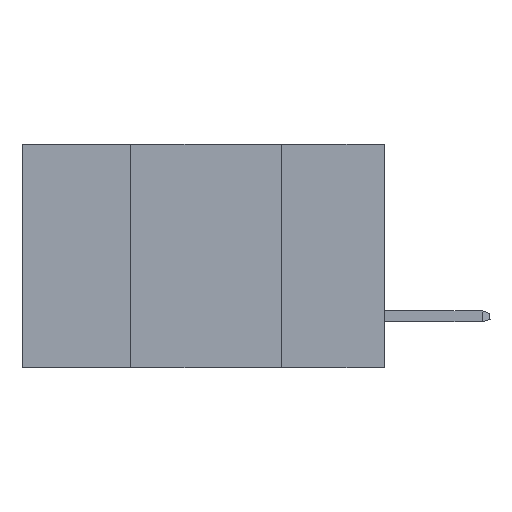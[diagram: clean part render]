
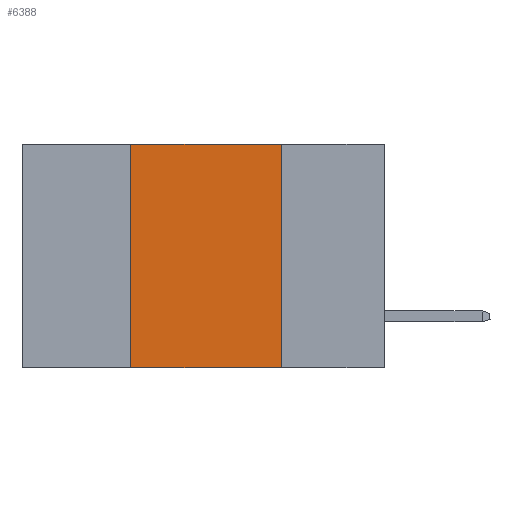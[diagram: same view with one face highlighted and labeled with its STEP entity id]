
A CAD part, left-side view. The second image highlights one B-rep face of the part: STEP entity #6388.
In plain terms, the highlighted planar face has unit normal (-1, 0, 0).
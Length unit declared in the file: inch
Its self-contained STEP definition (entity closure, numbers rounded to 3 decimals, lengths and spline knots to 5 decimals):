
#297 = VERTEX_POINT ( 'NONE', #6167 ) ;
#317 = LINE ( 'NONE', #12907, #29280 ) ;
#359 = DIRECTION ( 'NONE',  ( 0., 0., -1. ) ) ;
#3723 = EDGE_CURVE ( 'NONE', #297, #7186, #22911, .T. ) ;
#4326 = LINE ( 'NONE', #20937, #27781 ) ;
#5648 = ORIENTED_EDGE ( 'NONE', *, *, #17468, .F. ) ;
#5982 = ORIENTED_EDGE ( 'NONE', *, *, #3723, .F. ) ;
#6167 = CARTESIAN_POINT ( 'NONE',  ( 0., 0.42, 0. ) ) ;
#6230 = CARTESIAN_POINT ( 'NONE',  ( 0., 0.17, 0. ) ) ;
#6388 = ADVANCED_FACE ( 'NONE', ( #8823 ), #24045, .F. ) ;
#6998 = CARTESIAN_POINT ( 'NONE',  ( 0., 0.42, 0. ) ) ;
#7186 = VERTEX_POINT ( 'NONE', #6230 ) ;
#8091 = LINE ( 'NONE', #6998, #20207 ) ;
#8315 = EDGE_CURVE ( 'NONE', #20299, #24931, #317, .T. ) ;
#8823 = FACE_OUTER_BOUND ( 'NONE', #10262, .T. ) ;
#9251 = DIRECTION ( 'NONE',  ( 0., 0., 1. ) ) ;
#10262 = EDGE_LOOP ( 'NONE', ( #5648, #5982, #23977, #25939 ) ) ;
#10720 = VECTOR ( 'NONE', #26289, 39.37008 ) ;
#12516 = DIRECTION ( 'NONE',  ( 0., -1., 0. ) ) ;
#12907 = CARTESIAN_POINT ( 'NONE',  ( 0., 0.6, -0.37 ) ) ;
#14380 = EDGE_CURVE ( 'NONE', #20299, #297, #8091, .T. ) ;
#17468 = EDGE_CURVE ( 'NONE', #7186, #24931, #4326, .T. ) ;
#20207 = VECTOR ( 'NONE', #9251, 39.37008 ) ;
#20299 = VERTEX_POINT ( 'NONE', #26539 ) ;
#20937 = CARTESIAN_POINT ( 'NONE',  ( 0., 0.17, 0. ) ) ;
#22911 = LINE ( 'NONE', #27964, #10720 ) ;
#23977 = ORIENTED_EDGE ( 'NONE', *, *, #14380, .F. ) ;
#24045 = PLANE ( 'NONE',  #28192 ) ;
#24217 = DIRECTION ( 'NONE',  ( 0., 0., -1. ) ) ;
#24672 = DIRECTION ( 'NONE',  ( 1., 0., 0. ) ) ;
#24700 = CARTESIAN_POINT ( 'NONE',  ( 0., 0.6, 0. ) ) ;
#24931 = VERTEX_POINT ( 'NONE', #27484 ) ;
#25939 = ORIENTED_EDGE ( 'NONE', *, *, #8315, .T. ) ;
#26289 = DIRECTION ( 'NONE',  ( 0., -1., 0. ) ) ;
#26539 = CARTESIAN_POINT ( 'NONE',  ( 0., 0.42, -0.37 ) ) ;
#27484 = CARTESIAN_POINT ( 'NONE',  ( 0., 0.17, -0.37 ) ) ;
#27781 = VECTOR ( 'NONE', #359, 39.37008 ) ;
#27964 = CARTESIAN_POINT ( 'NONE',  ( 0., 0.6, 0. ) ) ;
#28192 = AXIS2_PLACEMENT_3D ( 'NONE', #24700, #24672, #24217 ) ;
#29280 = VECTOR ( 'NONE', #12516, 39.37008 ) ;
